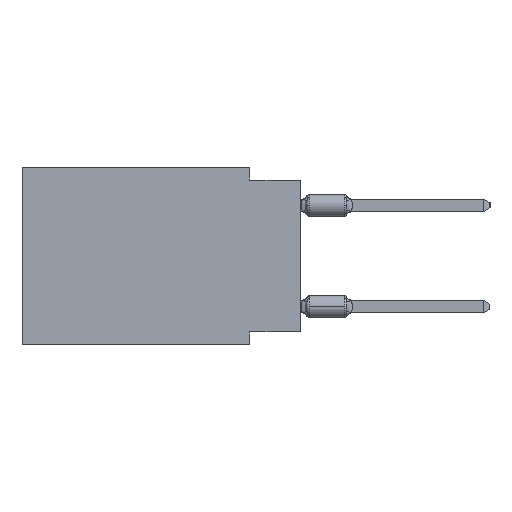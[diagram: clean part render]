
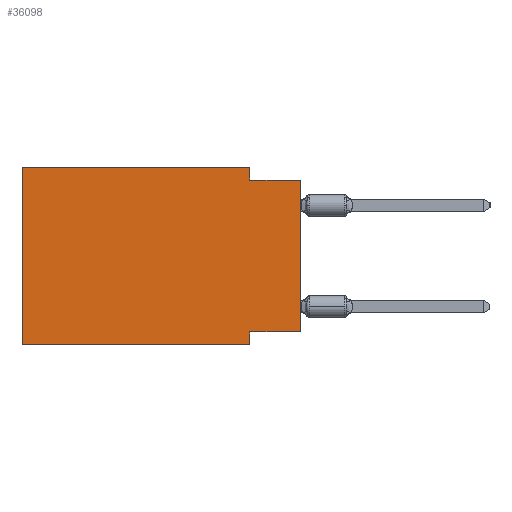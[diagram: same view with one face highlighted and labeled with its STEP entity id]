
A CAD part, left-side view. The second image highlights one B-rep face of the part: STEP entity #36098.
In plain terms, the highlighted planar face has unit normal (-1, 0, 0).
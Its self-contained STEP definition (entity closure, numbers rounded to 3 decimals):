
#1188 = ORIENTED_EDGE ( 'NONE', *, *, #59497, .T. ) ;
#1499 = PLANE ( 'NONE',  #61051 ) ;
#2368 = LINE ( 'NONE', #20468, #39475 ) ;
#2548 = DIRECTION ( 'NONE',  ( 0., -1., 0. ) ) ;
#3186 = VECTOR ( 'NONE', #42860, 1000. ) ;
#3521 = VECTOR ( 'NONE', #7240, 1000. ) ;
#3536 = LINE ( 'NONE', #34185, #41042 ) ;
#3793 = EDGE_CURVE ( 'NONE', #44724, #11164, #37019, .T. ) ;
#3843 = CARTESIAN_POINT ( 'NONE',  ( 0., 2.54, -8.255 ) ) ;
#4500 = DIRECTION ( 'NONE',  ( 0., 0., -1. ) ) ;
#5048 = DIRECTION ( 'NONE',  ( 0., 0., -1. ) ) ;
#5307 = ORIENTED_EDGE ( 'NONE', *, *, #35775, .F. ) ;
#7120 = LINE ( 'NONE', #7451, #3186 ) ;
#7240 = DIRECTION ( 'NONE',  ( 0., -1., 0. ) ) ;
#7451 = CARTESIAN_POINT ( 'NONE',  ( 0., 0., 0. ) ) ;
#8871 = LINE ( 'NONE', #13049, #60771 ) ;
#9213 = DIRECTION ( 'NONE',  ( 0., 1., 0. ) ) ;
#9746 = VERTEX_POINT ( 'NONE', #53366 ) ;
#10003 = ORIENTED_EDGE ( 'NONE', *, *, #25912, .F. ) ;
#11164 = VERTEX_POINT ( 'NONE', #40374 ) ;
#11901 = VERTEX_POINT ( 'NONE', #23568 ) ;
#13049 = CARTESIAN_POINT ( 'NONE',  ( 0., 0., -8.255 ) ) ;
#17550 = VECTOR ( 'NONE', #27781, 1000. ) ;
#18028 = EDGE_CURVE ( 'NONE', #27761, #45560, #8871, .T. ) ;
#20468 = CARTESIAN_POINT ( 'NONE',  ( 0., 2.54, -8.89 ) ) ;
#20543 = CARTESIAN_POINT ( 'NONE',  ( 0., 13.97, -8.89 ) ) ;
#21258 = ORIENTED_EDGE ( 'NONE', *, *, #3793, .F. ) ;
#21541 = DIRECTION ( 'NONE',  ( 1., 0., 0. ) ) ;
#23568 = CARTESIAN_POINT ( 'NONE',  ( 0., 13.97, 0. ) ) ;
#24005 = ORIENTED_EDGE ( 'NONE', *, *, #28103, .F. ) ;
#25912 = EDGE_CURVE ( 'NONE', #11164, #30457, #54541, .T. ) ;
#26018 = ORIENTED_EDGE ( 'NONE', *, *, #39862, .F. ) ;
#27761 = VERTEX_POINT ( 'NONE', #35740 ) ;
#27781 = DIRECTION ( 'NONE',  ( 0., 0., 1. ) ) ;
#28103 = EDGE_CURVE ( 'NONE', #45560, #9746, #2368, .T. ) ;
#30457 = VERTEX_POINT ( 'NONE', #37991 ) ;
#34185 = CARTESIAN_POINT ( 'NONE',  ( 0., 13.97, -8.89 ) ) ;
#35740 = CARTESIAN_POINT ( 'NONE',  ( 0., 0., -8.255 ) ) ;
#35775 = EDGE_CURVE ( 'NONE', #62433, #11901, #59484, .T. ) ;
#36098 = ADVANCED_FACE ( 'NONE', ( #41654 ), #1499, .F. ) ;
#36866 = CARTESIAN_POINT ( 'NONE',  ( 0., 13.97, 0. ) ) ;
#37019 = LINE ( 'NONE', #57812, #59468 ) ;
#37991 = CARTESIAN_POINT ( 'NONE',  ( 0., 0., -0.635 ) ) ;
#39475 = VECTOR ( 'NONE', #4500, 1000. ) ;
#39862 = EDGE_CURVE ( 'NONE', #11901, #44724, #56993, .T. ) ;
#40374 = CARTESIAN_POINT ( 'NONE',  ( 0., 2.54, -0.635 ) ) ;
#41042 = VECTOR ( 'NONE', #2548, 1000. ) ;
#41654 = FACE_OUTER_BOUND ( 'NONE', #56530, .T. ) ;
#41698 = EDGE_CURVE ( 'NONE', #27761, #30457, #7120, .T. ) ;
#41985 = DIRECTION ( 'NONE',  ( 0., -1., 0. ) ) ;
#41988 = DIRECTION ( 'NONE',  ( 0., 0., -1. ) ) ;
#42322 = CARTESIAN_POINT ( 'NONE',  ( 0., 13.97, 0. ) ) ;
#42860 = DIRECTION ( 'NONE',  ( 0., 0., 1. ) ) ;
#44724 = VERTEX_POINT ( 'NONE', #61526 ) ;
#45560 = VERTEX_POINT ( 'NONE', #3843 ) ;
#48424 = CARTESIAN_POINT ( 'NONE',  ( 0., 0., -0.635 ) ) ;
#53030 = ORIENTED_EDGE ( 'NONE', *, *, #18028, .F. ) ;
#53366 = CARTESIAN_POINT ( 'NONE',  ( 0., 2.54, -8.89 ) ) ;
#53692 = CARTESIAN_POINT ( 'NONE',  ( 0., 13.97, 0. ) ) ;
#54541 = LINE ( 'NONE', #48424, #3521 ) ;
#56530 = EDGE_LOOP ( 'NONE', ( #61198, #10003, #21258, #26018, #5307, #1188, #24005, #53030 ) ) ;
#56993 = LINE ( 'NONE', #42322, #65340 ) ;
#57812 = CARTESIAN_POINT ( 'NONE',  ( 0., 2.54, 0. ) ) ;
#59468 = VECTOR ( 'NONE', #5048, 1000. ) ;
#59484 = LINE ( 'NONE', #53692, #17550 ) ;
#59497 = EDGE_CURVE ( 'NONE', #62433, #9746, #3536, .T. ) ;
#60771 = VECTOR ( 'NONE', #9213, 1000. ) ;
#61051 = AXIS2_PLACEMENT_3D ( 'NONE', #36866, #21541, #41988 ) ;
#61198 = ORIENTED_EDGE ( 'NONE', *, *, #41698, .T. ) ;
#61526 = CARTESIAN_POINT ( 'NONE',  ( 0., 2.54, 0. ) ) ;
#62433 = VERTEX_POINT ( 'NONE', #20543 ) ;
#65340 = VECTOR ( 'NONE', #41985, 1000. ) ;
